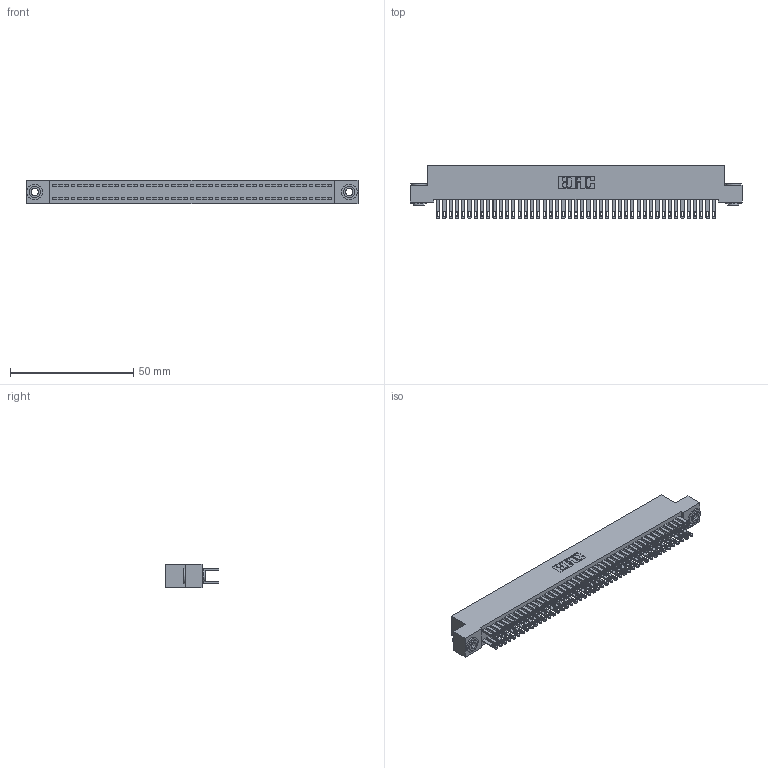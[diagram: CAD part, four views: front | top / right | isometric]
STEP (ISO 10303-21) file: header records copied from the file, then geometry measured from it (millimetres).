
FILE_DESCRIPTION (( 'STEP AP203' ), '1' );
FILE_NAME ('342-090-500-203.STEP', '2018-08-14T00:50:00', ( '' ), ( '' ), 'SwSTEP 2.0', 'SolidWorks 2016', '' );
FILE_SCHEMA (( 'CONFIG_CONTROL_DESIGN' ));
Length unit declared in the file: inch
Products named in the file (4): 342 Part_.156 TH; 345-292-001_345-293-100; 342-250-002_345-250-002-102; 342-090-500-203
Assembly tree (93 placements, depth 2):
  342-090-500-203
    342 Part_.156 TH
    345-292-001_345-293-100  x90
    342-250-002_345-250-002-102  x2
Bounding box: 134.62 x 21.85 x 9.4 mm (x, y, z)
Volume: 12407.6 mm3; surface area: 21346.2 mm2
Topology: 93 solids, 93 shells, 4468 faces, 13605 edges, 9066 vertices
Faces by surface type: plane 2776, cylinder 1684, cone 8
Entity records: 29010 total; most frequent: CARTESIAN_POINT 4777, ORIENTED_EDGE 4706, DIRECTION 4111, EDGE_CURVE 2353, VECTOR 2197, LINE 2197, VERTEX_POINT 1566, AXIS2_PLACEMENT_3D 957
